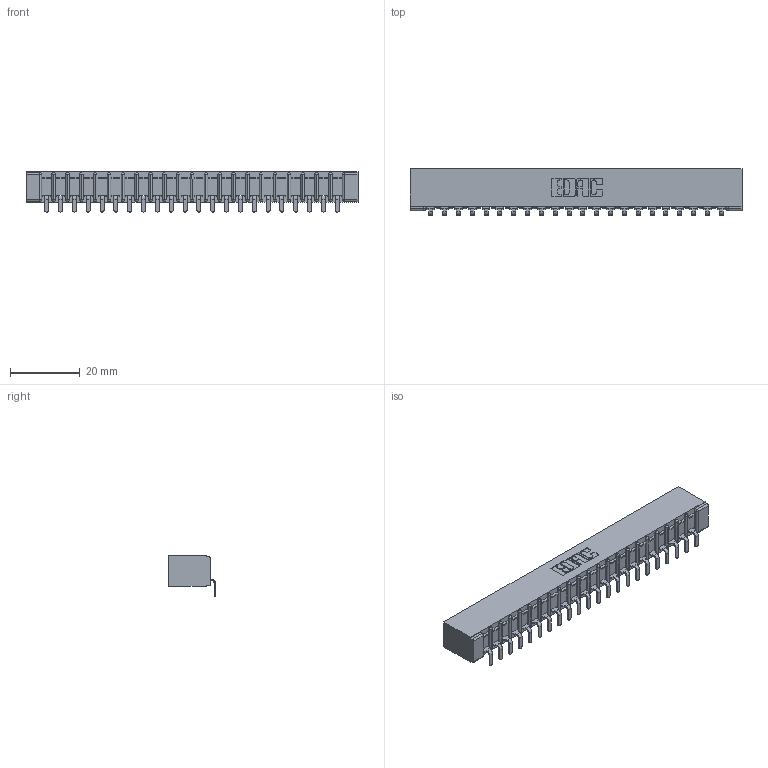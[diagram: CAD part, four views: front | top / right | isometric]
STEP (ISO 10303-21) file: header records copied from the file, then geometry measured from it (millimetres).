
FILE_DESCRIPTION (( 'STEP AP203' ), '1' );
FILE_NAME ('307-022-553-101.STEP', '2018-08-04T03:46:40', ( '' ), ( '' ), 'SwSTEP 2.0', 'SolidWorks 2016', '' );
FILE_SCHEMA (( 'CONFIG_CONTROL_DESIGN' ));
Length unit declared in the file: inch
Products named in the file (3): 307 Part_No Mounting Lugs; 307-290-002_553; 307-022-553-101
Assembly tree (23 placements, depth 2):
  307-022-553-101
    307 Part_No Mounting Lugs
    307-290-002_553  x22
Bounding box: 95.05 x 13.32 x 11.51 mm (x, y, z)
Volume: 6517 mm3; surface area: 12367.2 mm2
Topology: 23 solids, 23 shells, 1849 faces, 5667 edges, 3714 vertices
Faces by surface type: plane 1100, cylinder 703, sphere 46
Entity records: 21902 total; most frequent: CARTESIAN_POINT 3692, ORIENTED_EDGE 3682, DIRECTION 3595, EDGE_CURVE 1841, LINE 1401, VECTOR 1401, VERTEX_POINT 1194, AXIS2_PLACEMENT_3D 1097
